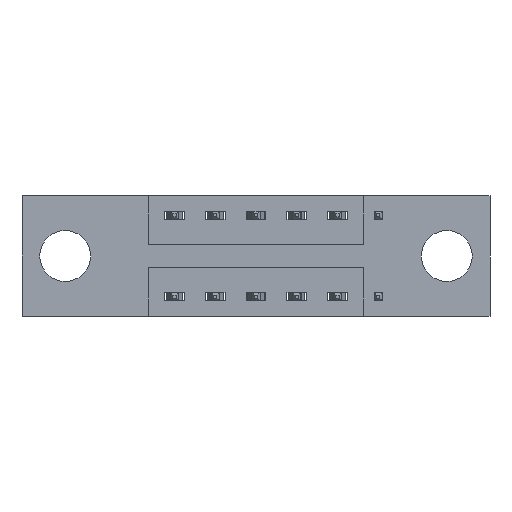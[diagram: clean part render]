
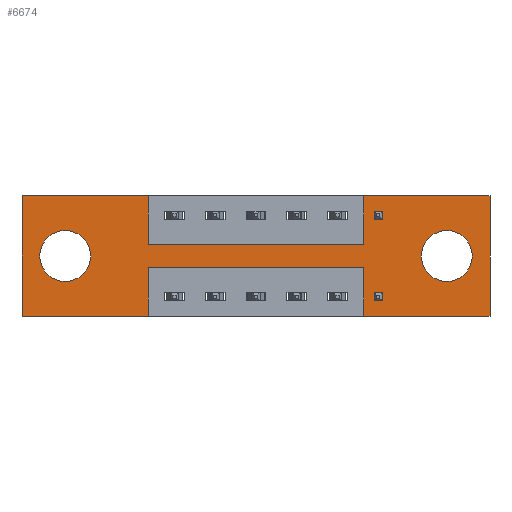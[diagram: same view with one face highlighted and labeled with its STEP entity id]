
A CAD part, front view. The second image highlights one B-rep face of the part: STEP entity #6674.
In plain terms, the highlighted planar face has unit normal (0, -1, 0).
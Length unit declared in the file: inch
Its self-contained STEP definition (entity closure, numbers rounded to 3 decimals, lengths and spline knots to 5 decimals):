
#1 = CARTESIAN_POINT ( 'NONE',  ( 0.1325, 0., -0.185 ) ) ;
#120 = LINE ( 'NONE', #6161, #7895 ) ;
#130 = CARTESIAN_POINT ( 'NONE',  ( 1.0475, 0., 0. ) ) ;
#158 = VERTEX_POINT ( 'NONE', #215 ) ;
#174 = CARTESIAN_POINT ( 'NONE',  ( 0.3875, 0., -0.22 ) ) ;
#215 = CARTESIAN_POINT ( 'NONE',  ( 0.1325, 0., -0.263 ) ) ;
#247 = CARTESIAN_POINT ( 'NONE',  ( 1.0475, 0., -0.22 ) ) ;
#292 = VECTOR ( 'NONE', #957, 39.37008 ) ;
#451 = LINE ( 'NONE', #5252, #4660 ) ;
#497 = VECTOR ( 'NONE', #5572, 39.37008 ) ;
#513 = VECTOR ( 'NONE', #742, 39.37008 ) ;
#553 = DIRECTION ( 'NONE',  ( 0., 0., -1. ) ) ;
#596 = DIRECTION ( 'NONE',  ( 1., 0., 0. ) ) ;
#634 = DIRECTION ( 'NONE',  ( 1., 0., 0. ) ) ;
#666 = EDGE_CURVE ( 'NONE', #1883, #3743, #5725, .T. ) ;
#742 = DIRECTION ( 'NONE',  ( -1., 0., 0. ) ) ;
#783 = VECTOR ( 'NONE', #596, 39.37008 ) ;
#880 = CARTESIAN_POINT ( 'NONE',  ( 1.0475, 0., -0.15 ) ) ;
#931 = DIRECTION ( 'NONE',  ( 0., 0., 1. ) ) ;
#957 = DIRECTION ( 'NONE',  ( -1., 0., 0. ) ) ;
#960 = VECTOR ( 'NONE', #553, 39.37008 ) ;
#966 = LINE ( 'NONE', #5185, #4358 ) ;
#1003 = ORIENTED_EDGE ( 'NONE', *, *, #8142, .F. ) ;
#1049 = ORIENTED_EDGE ( 'NONE', *, *, #4044, .F. ) ;
#1093 = CARTESIAN_POINT ( 'NONE',  ( 0., 0., -0.37 ) ) ;
#1196 = CARTESIAN_POINT ( 'NONE',  ( 1.3025, 0., -0.185 ) ) ;
#1264 = CARTESIAN_POINT ( 'NONE',  ( 0.1325, 0., -0.185 ) ) ;
#1442 = DIRECTION ( 'NONE',  ( 0., 0., 1. ) ) ;
#1597 = LINE ( 'NONE', #6532, #6899 ) ;
#1603 = LINE ( 'NONE', #7013, #8190 ) ;
#1611 = LINE ( 'NONE', #6982, #2257 ) ;
#1654 = CARTESIAN_POINT ( 'NONE',  ( 0., 0., -0.37 ) ) ;
#1680 = VERTEX_POINT ( 'NONE', #8245 ) ;
#1883 = VERTEX_POINT ( 'NONE', #5222 ) ;
#1922 = CIRCLE ( 'NONE', #6891, 0.078 ) ;
#2230 = DIRECTION ( 'NONE',  ( 0., -1., 0. ) ) ;
#2251 = CARTESIAN_POINT ( 'NONE',  ( 1.435, 0., -0.37 ) ) ;
#2257 = VECTOR ( 'NONE', #5531, 39.37008 ) ;
#2427 = LINE ( 'NONE', #5279, #783 ) ;
#2482 = EDGE_CURVE ( 'NONE', #6620, #7104, #2427, .T. ) ;
#2547 = CARTESIAN_POINT ( 'NONE',  ( 0.3875, 0., -0.37 ) ) ;
#2550 = VERTEX_POINT ( 'NONE', #8413 ) ;
#2569 = EDGE_CURVE ( 'NONE', #4256, #4537, #966, .T. ) ;
#2618 = VERTEX_POINT ( 'NONE', #1093 ) ;
#2632 = EDGE_CURVE ( 'NONE', #2550, #4480, #6378, .T. ) ;
#2641 = LINE ( 'NONE', #3180, #960 ) ;
#2668 = DIRECTION ( 'NONE',  ( 0., 1., 0. ) ) ;
#2693 = CARTESIAN_POINT ( 'NONE',  ( 1.0475, 0., 0. ) ) ;
#2811 = VERTEX_POINT ( 'NONE', #2693 ) ;
#3180 = CARTESIAN_POINT ( 'NONE',  ( 0.3875, 0., -0.37 ) ) ;
#3449 = EDGE_CURVE ( 'NONE', #5105, #158, #4940, .T. ) ;
#3451 = EDGE_LOOP ( 'NONE', ( #5390, #8528 ) ) ;
#3493 = DIRECTION ( 'NONE',  ( 0., 0., 1. ) ) ;
#3534 = CIRCLE ( 'NONE', #5382, 0.078 ) ;
#3705 = CARTESIAN_POINT ( 'NONE',  ( 1.435, 0., 0. ) ) ;
#3743 = VERTEX_POINT ( 'NONE', #3931 ) ;
#3786 = DIRECTION ( 'NONE',  ( 0., 0., 1. ) ) ;
#3926 = DIRECTION ( 'NONE',  ( 0., 0., -1. ) ) ;
#3931 = CARTESIAN_POINT ( 'NONE',  ( 1.3025, 0., -0.107 ) ) ;
#4039 = ORIENTED_EDGE ( 'NONE', *, *, #7098, .F. ) ;
#4044 = EDGE_CURVE ( 'NONE', #2618, #6620, #1597, .T. ) ;
#4091 = ORIENTED_EDGE ( 'NONE', *, *, #6117, .F. ) ;
#4166 = EDGE_CURVE ( 'NONE', #4480, #8506, #451, .T. ) ;
#4192 = CARTESIAN_POINT ( 'NONE',  ( 0.3875, 0., -0.15 ) ) ;
#4256 = VERTEX_POINT ( 'NONE', #4192 ) ;
#4348 = CARTESIAN_POINT ( 'NONE',  ( 1.0475, 0., -0.37 ) ) ;
#4358 = VECTOR ( 'NONE', #5813, 39.37008 ) ;
#4395 = DIRECTION ( 'NONE',  ( 0., 0., -1. ) ) ;
#4440 = ORIENTED_EDGE ( 'NONE', *, *, #5032, .T. ) ;
#4471 = DIRECTION ( 'NONE',  ( 0., 1., 0. ) ) ;
#4480 = VERTEX_POINT ( 'NONE', #2251 ) ;
#4537 = VERTEX_POINT ( 'NONE', #880 ) ;
#4660 = VECTOR ( 'NONE', #5380, 39.37008 ) ;
#4663 = DIRECTION ( 'NONE',  ( 0., 1., 0. ) ) ;
#4729 = EDGE_CURVE ( 'NONE', #5299, #1680, #6171, .T. ) ;
#4764 = ORIENTED_EDGE ( 'NONE', *, *, #4166, .F. ) ;
#4940 = CIRCLE ( 'NONE', #8158, 0.078 ) ;
#5010 = FACE_BOUND ( 'NONE', #5024, .T. ) ;
#5024 = EDGE_LOOP ( 'NONE', ( #7577, #4440 ) ) ;
#5032 = EDGE_CURVE ( 'NONE', #158, #5105, #1922, .T. ) ;
#5105 = VERTEX_POINT ( 'NONE', #8487 ) ;
#5185 = CARTESIAN_POINT ( 'NONE',  ( 0.3875, 0., -0.15 ) ) ;
#5222 = CARTESIAN_POINT ( 'NONE',  ( 1.3025, 0., -0.263 ) ) ;
#5229 = DIRECTION ( 'NONE',  ( 0., 0., 1. ) ) ;
#5252 = CARTESIAN_POINT ( 'NONE',  ( 0., 0., -0.37 ) ) ;
#5279 = CARTESIAN_POINT ( 'NONE',  ( 0., 0., 0. ) ) ;
#5299 = VERTEX_POINT ( 'NONE', #247 ) ;
#5380 = DIRECTION ( 'NONE',  ( -1., 0., 0. ) ) ;
#5382 = AXIS2_PLACEMENT_3D ( 'NONE', #8231, #2668, #7526 ) ;
#5390 = ORIENTED_EDGE ( 'NONE', *, *, #7129, .T. ) ;
#5417 = EDGE_LOOP ( 'NONE', ( #7731, #8097, #4039, #4764, #8006, #7680, #4091, #8764, #5834, #6260, #1049, #1003 ) ) ;
#5531 = DIRECTION ( 'NONE',  ( 0., 0., -1. ) ) ;
#5572 = DIRECTION ( 'NONE',  ( 0., 0., -1. ) ) ;
#5617 = PLANE ( 'NONE',  #8046 ) ;
#5677 = CARTESIAN_POINT ( 'NONE',  ( 0., 0., -0.37 ) ) ;
#5706 = CARTESIAN_POINT ( 'NONE',  ( 0.3875, 0., 0. ) ) ;
#5713 = CARTESIAN_POINT ( 'NONE',  ( 0., 0., 0. ) ) ;
#5725 = CIRCLE ( 'NONE', #7256, 0.078 ) ;
#5813 = DIRECTION ( 'NONE',  ( 1., 0., 0. ) ) ;
#5834 = ORIENTED_EDGE ( 'NONE', *, *, #8385, .F. ) ;
#6117 = EDGE_CURVE ( 'NONE', #4537, #2811, #8143, .T. ) ;
#6161 = CARTESIAN_POINT ( 'NONE',  ( 0., 0., 0. ) ) ;
#6171 = LINE ( 'NONE', #174, #513 ) ;
#6260 = ORIENTED_EDGE ( 'NONE', *, *, #2482, .F. ) ;
#6341 = FACE_OUTER_BOUND ( 'NONE', #5417, .T. ) ;
#6346 = EDGE_CURVE ( 'NONE', #1680, #6848, #2641, .T. ) ;
#6378 = LINE ( 'NONE', #3705, #497 ) ;
#6498 = EDGE_CURVE ( 'NONE', #2811, #2550, #120, .T. ) ;
#6532 = CARTESIAN_POINT ( 'NONE',  ( 0., 0., 0. ) ) ;
#6620 = VERTEX_POINT ( 'NONE', #5713 ) ;
#6674 = ADVANCED_FACE ( 'NONE', ( #7109, #5010, #6341 ), #5617, .T. ) ;
#6848 = VERTEX_POINT ( 'NONE', #2547 ) ;
#6891 = AXIS2_PLACEMENT_3D ( 'NONE', #1264, #4663, #5229 ) ;
#6899 = VECTOR ( 'NONE', #3786, 39.37008 ) ;
#6982 = CARTESIAN_POINT ( 'NONE',  ( 0.3875, 0., 0. ) ) ;
#7013 = CARTESIAN_POINT ( 'NONE',  ( 1.0475, 0., -0.37 ) ) ;
#7079 = LINE ( 'NONE', #5677, #292 ) ;
#7098 = EDGE_CURVE ( 'NONE', #8506, #5299, #1603, .T. ) ;
#7104 = VERTEX_POINT ( 'NONE', #5706 ) ;
#7109 = FACE_BOUND ( 'NONE', #3451, .T. ) ;
#7129 = EDGE_CURVE ( 'NONE', #3743, #1883, #3534, .T. ) ;
#7174 = VECTOR ( 'NONE', #1442, 39.37008 ) ;
#7256 = AXIS2_PLACEMENT_3D ( 'NONE', #1196, #4471, #3926 ) ;
#7526 = DIRECTION ( 'NONE',  ( 0., 0., -1. ) ) ;
#7577 = ORIENTED_EDGE ( 'NONE', *, *, #3449, .T. ) ;
#7680 = ORIENTED_EDGE ( 'NONE', *, *, #6498, .F. ) ;
#7731 = ORIENTED_EDGE ( 'NONE', *, *, #6346, .F. ) ;
#7895 = VECTOR ( 'NONE', #634, 39.37008 ) ;
#8006 = ORIENTED_EDGE ( 'NONE', *, *, #2632, .F. ) ;
#8046 = AXIS2_PLACEMENT_3D ( 'NONE', #1654, #2230, #4395 ) ;
#8097 = ORIENTED_EDGE ( 'NONE', *, *, #4729, .F. ) ;
#8139 = DIRECTION ( 'NONE',  ( 0., 1., 0. ) ) ;
#8142 = EDGE_CURVE ( 'NONE', #6848, #2618, #7079, .T. ) ;
#8143 = LINE ( 'NONE', #130, #7174 ) ;
#8158 = AXIS2_PLACEMENT_3D ( 'NONE', #1, #8139, #3493 ) ;
#8190 = VECTOR ( 'NONE', #931, 39.37008 ) ;
#8231 = CARTESIAN_POINT ( 'NONE',  ( 1.3025, 0., -0.185 ) ) ;
#8245 = CARTESIAN_POINT ( 'NONE',  ( 0.3875, 0., -0.22 ) ) ;
#8385 = EDGE_CURVE ( 'NONE', #7104, #4256, #1611, .T. ) ;
#8413 = CARTESIAN_POINT ( 'NONE',  ( 1.435, 0., 0. ) ) ;
#8487 = CARTESIAN_POINT ( 'NONE',  ( 0.1325, 0., -0.107 ) ) ;
#8506 = VERTEX_POINT ( 'NONE', #4348 ) ;
#8528 = ORIENTED_EDGE ( 'NONE', *, *, #666, .T. ) ;
#8764 = ORIENTED_EDGE ( 'NONE', *, *, #2569, .F. ) ;
